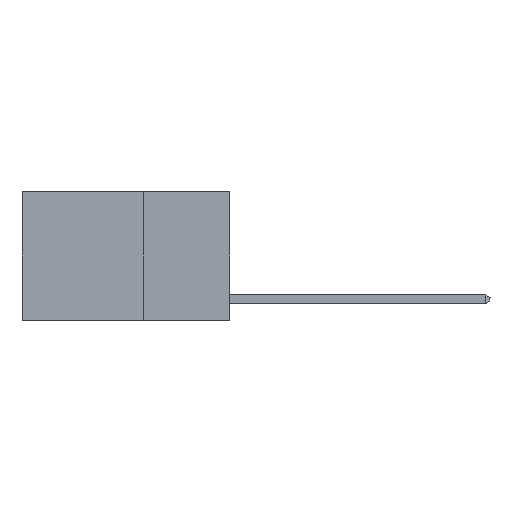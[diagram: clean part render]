
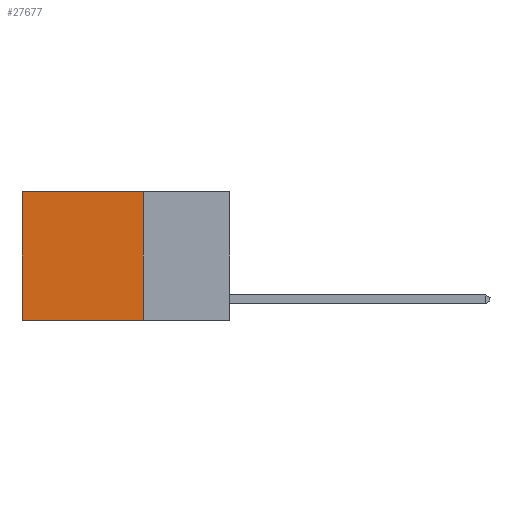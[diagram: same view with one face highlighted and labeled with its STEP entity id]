
A CAD part, left-side view. The second image highlights one B-rep face of the part: STEP entity #27677.
In plain terms, the highlighted planar face has unit normal (-1, 0, 0).
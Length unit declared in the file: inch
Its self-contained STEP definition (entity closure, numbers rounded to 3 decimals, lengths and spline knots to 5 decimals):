
#245 = VERTEX_POINT ( 'NONE', #11128 ) ;
#389 = VERTEX_POINT ( 'NONE', #27243 ) ;
#3430 = DIRECTION ( 'NONE',  ( 0., 1., 0. ) ) ;
#3975 = DIRECTION ( 'NONE',  ( 1., 0., 0. ) ) ;
#6181 = VECTOR ( 'NONE', #20122, 39.37008 ) ;
#6265 = VECTOR ( 'NONE', #3430, 39.37008 ) ;
#7514 = VERTEX_POINT ( 'NONE', #16317 ) ;
#8048 = LINE ( 'NONE', #28066, #6265 ) ;
#8447 = FACE_OUTER_BOUND ( 'NONE', #19291, .T. ) ;
#8696 = DIRECTION ( 'NONE',  ( 0., 0., -1. ) ) ;
#8890 = EDGE_CURVE ( 'NONE', #17157, #245, #18651, .T. ) ;
#10076 = EDGE_CURVE ( 'NONE', #17157, #389, #19577, .T. ) ;
#10435 = LINE ( 'NONE', #23834, #18782 ) ;
#11126 = AXIS2_PLACEMENT_3D ( 'NONE', #16969, #3975, #17263 ) ;
#11128 = CARTESIAN_POINT ( 'NONE',  ( 0.2625, 0.6, 0. ) ) ;
#12305 = EDGE_CURVE ( 'NONE', #389, #7514, #8048, .T. ) ;
#13346 = ORIENTED_EDGE ( 'NONE', *, *, #21359, .T. ) ;
#13382 = ORIENTED_EDGE ( 'NONE', *, *, #8890, .T. ) ;
#15871 = CARTESIAN_POINT ( 'NONE',  ( 0.2625, 0.25, 0. ) ) ;
#16317 = CARTESIAN_POINT ( 'NONE',  ( 0.2625, 0.6, -0.37 ) ) ;
#16677 = ORIENTED_EDGE ( 'NONE', *, *, #10076, .F. ) ;
#16768 = CARTESIAN_POINT ( 'NONE',  ( 0.2625, 0.25, 0. ) ) ;
#16969 = CARTESIAN_POINT ( 'NONE',  ( 0.2625, 0.25, 0. ) ) ;
#17157 = VERTEX_POINT ( 'NONE', #15871 ) ;
#17263 = DIRECTION ( 'NONE',  ( 0., 0., -1. ) ) ;
#18651 = LINE ( 'NONE', #16768, #19991 ) ;
#18782 = VECTOR ( 'NONE', #8696, 39.37008 ) ;
#19291 = EDGE_LOOP ( 'NONE', ( #13346, #20617, #16677, #13382 ) ) ;
#19577 = LINE ( 'NONE', #22288, #6181 ) ;
#19991 = VECTOR ( 'NONE', #27272, 39.37008 ) ;
#20122 = DIRECTION ( 'NONE',  ( 0., 0., -1. ) ) ;
#20617 = ORIENTED_EDGE ( 'NONE', *, *, #12305, .F. ) ;
#21279 = PLANE ( 'NONE',  #11126 ) ;
#21359 = EDGE_CURVE ( 'NONE', #245, #7514, #10435, .T. ) ;
#22288 = CARTESIAN_POINT ( 'NONE',  ( 0.2625, 0.25, 0. ) ) ;
#23834 = CARTESIAN_POINT ( 'NONE',  ( 0.2625, 0.6, 0. ) ) ;
#27243 = CARTESIAN_POINT ( 'NONE',  ( 0.2625, 0.25, -0.37 ) ) ;
#27272 = DIRECTION ( 'NONE',  ( 0., 1., 0. ) ) ;
#27677 = ADVANCED_FACE ( 'NONE', ( #8447 ), #21279, .F. ) ;
#28066 = CARTESIAN_POINT ( 'NONE',  ( 0.2625, 0.25, -0.37 ) ) ;
